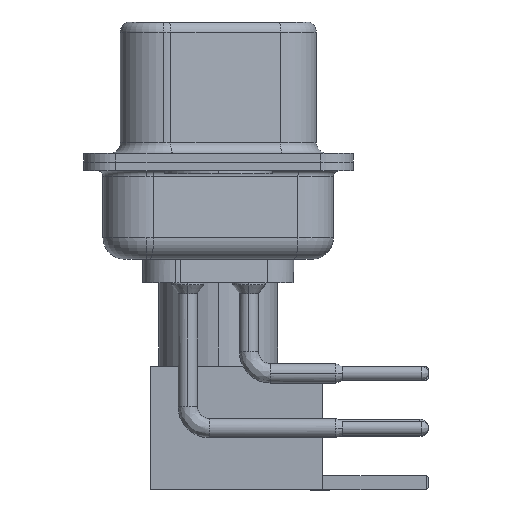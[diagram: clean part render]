
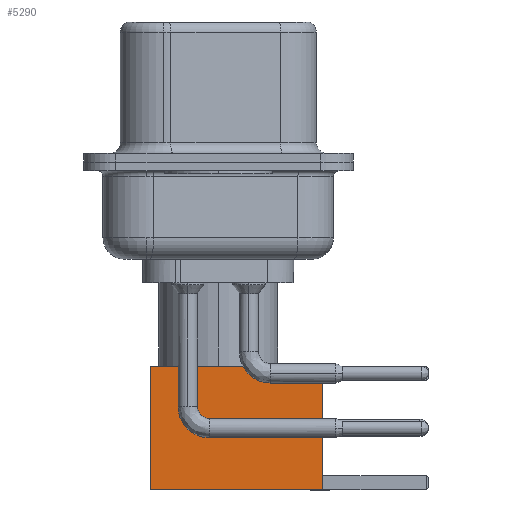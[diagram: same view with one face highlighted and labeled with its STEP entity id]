
A CAD part, left-side view. The second image highlights one B-rep face of the part: STEP entity #5290.
In plain terms, the highlighted face is planar.
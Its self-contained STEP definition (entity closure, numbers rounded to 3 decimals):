
#631 = CARTESIAN_POINT ( 'NONE',  ( 2.875, 2.875, 0. ) ) ;
#662 = EDGE_CURVE ( 'NONE', #18091, #12166, #7372, .T. ) ;
#771 = EDGE_LOOP ( 'NONE', ( #15364, #14729, #15446, #21229 ) ) ;
#933 = VECTOR ( 'NONE', #1018, 1000. ) ;
#1018 = DIRECTION ( 'NONE',  ( -1., 0., 0. ) ) ;
#1389 = CARTESIAN_POINT ( 'NONE',  ( 2.875, 2.875, 0. ) ) ;
#1397 = CARTESIAN_POINT ( 'NONE',  ( -2.875, 2.875, 0. ) ) ;
#3439 = VECTOR ( 'NONE', #11549, 1000. ) ;
#4044 = EDGE_CURVE ( 'NONE', #17011, #12166, #15677, .T. ) ;
#5290 = ADVANCED_FACE ( 'NONE', ( #8943 ), #9260, .T. ) ;
#5312 = CARTESIAN_POINT ( 'NONE',  ( -2.875, 2.875, 8. ) ) ;
#6334 = LINE ( 'NONE', #17966, #3439 ) ;
#7298 = DIRECTION ( 'NONE',  ( 0., 0., 1. ) ) ;
#7372 = LINE ( 'NONE', #12341, #21147 ) ;
#7429 = DIRECTION ( 'NONE',  ( 0., 0., -1. ) ) ;
#7653 = CARTESIAN_POINT ( 'NONE',  ( -2.875, 2.875, 0. ) ) ;
#8166 = VECTOR ( 'NONE', #7429, 1000. ) ;
#8943 = FACE_OUTER_BOUND ( 'NONE', #771, .T. ) ;
#9260 = PLANE ( 'NONE',  #17655 ) ;
#9323 = LINE ( 'NONE', #14796, #933 ) ;
#11549 = DIRECTION ( 'NONE',  ( 0., 0., -1. ) ) ;
#12166 = VERTEX_POINT ( 'NONE', #1397 ) ;
#12341 = CARTESIAN_POINT ( 'NONE',  ( 0., 2.875, 0. ) ) ;
#14729 = ORIENTED_EDGE ( 'NONE', *, *, #662, .T. ) ;
#14796 = CARTESIAN_POINT ( 'NONE',  ( 0., 2.875, 8. ) ) ;
#15364 = ORIENTED_EDGE ( 'NONE', *, *, #20868, .T. ) ;
#15370 = CARTESIAN_POINT ( 'NONE',  ( 2.875, 2.875, 8. ) ) ;
#15446 = ORIENTED_EDGE ( 'NONE', *, *, #4044, .F. ) ;
#15677 = LINE ( 'NONE', #7653, #8166 ) ;
#15869 = DIRECTION ( 'NONE',  ( 0., 1., 0. ) ) ;
#16153 = DIRECTION ( 'NONE',  ( -1., 0., 0. ) ) ;
#17011 = VERTEX_POINT ( 'NONE', #5312 ) ;
#17420 = VERTEX_POINT ( 'NONE', #15370 ) ;
#17655 = AXIS2_PLACEMENT_3D ( 'NONE', #631, #15869, #7298 ) ;
#17966 = CARTESIAN_POINT ( 'NONE',  ( 2.875, 2.875, 0. ) ) ;
#18091 = VERTEX_POINT ( 'NONE', #1389 ) ;
#19023 = EDGE_CURVE ( 'NONE', #17420, #17011, #9323, .T. ) ;
#20868 = EDGE_CURVE ( 'NONE', #17420, #18091, #6334, .T. ) ;
#21147 = VECTOR ( 'NONE', #16153, 1000. ) ;
#21229 = ORIENTED_EDGE ( 'NONE', *, *, #19023, .F. ) ;
